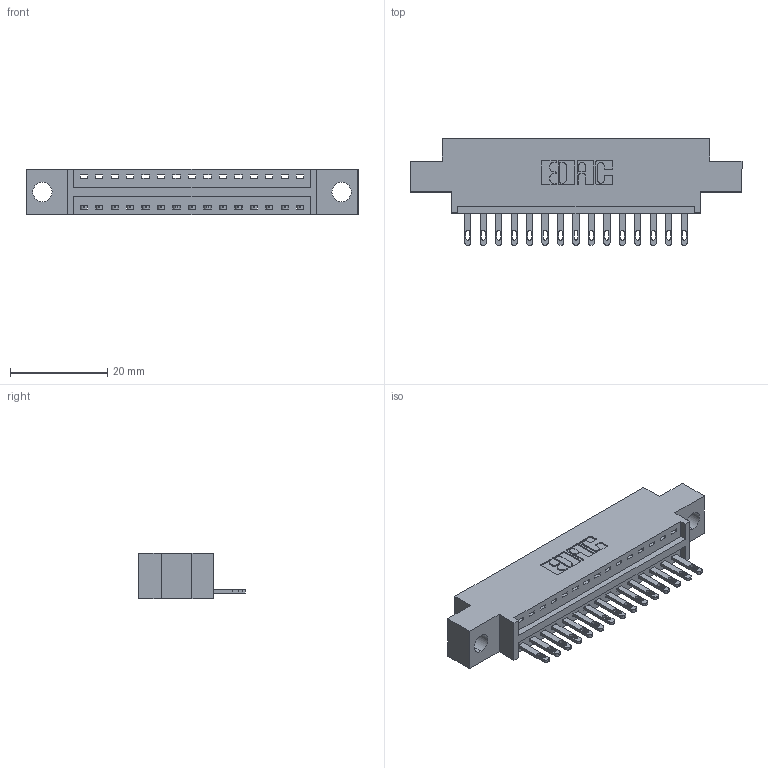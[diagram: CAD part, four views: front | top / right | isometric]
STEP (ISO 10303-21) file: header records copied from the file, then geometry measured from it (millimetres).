
FILE_DESCRIPTION (( 'STEP AP203' ), '1' );
FILE_NAME ('896-015-500-604.STEP', '2021-07-27T15:29:33', ( '' ), ( '' ), 'SwSTEP 2.0', 'SolidWorks 2020', '' );
FILE_SCHEMA (( 'CONFIG_CONTROL_DESIGN' ));
Length unit declared in the file: inch
Products named in the file (3): 345-292-001_345-293-100; 896-015-500-604; 846 Part_0.170 Offset - 0.156 Dia-TH
Assembly tree (16 placements, depth 2):
  896-015-500-604
    846 Part_0.170 Offset - 0.156 Dia-TH
    345-292-001_345-293-100  x15
Bounding box: 68.2 x 21.84 x 9.4 mm (x, y, z)
Volume: 6108.9 mm3; surface area: 7344.3 mm2
Topology: 16 solids, 16 shells, 936 faces, 2861 edges, 1906 vertices
Faces by surface type: plane 590, cylinder 346
Entity records: 13009 total; most frequent: CARTESIAN_POINT 2245, ORIENTED_EDGE 2194, DIRECTION 2015, EDGE_CURVE 1097, VECTOR 901, LINE 901, VERTEX_POINT 730, AXIS2_PLACEMENT_3D 557
